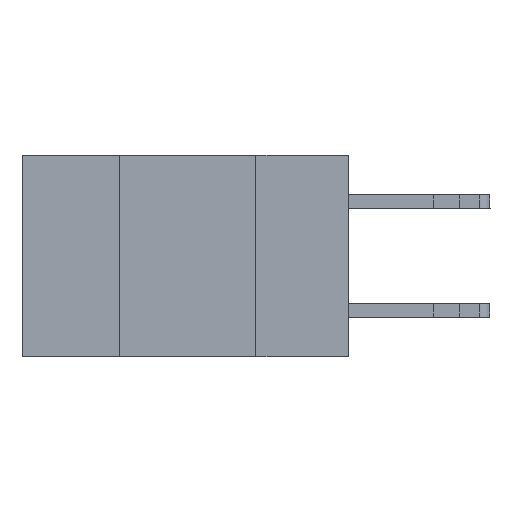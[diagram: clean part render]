
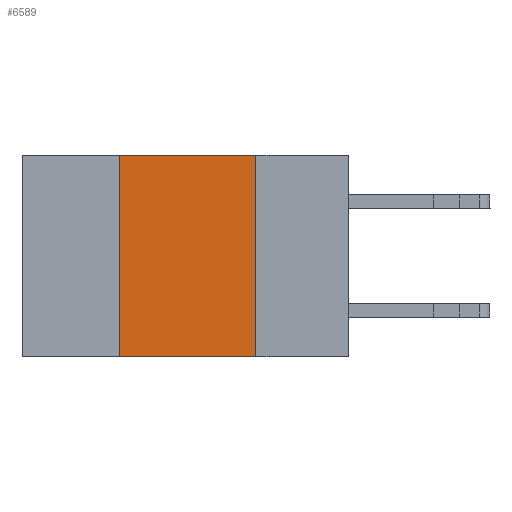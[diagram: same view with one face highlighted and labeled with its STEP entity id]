
A CAD part, left-side view. The second image highlights one B-rep face of the part: STEP entity #6589.
In plain terms, the highlighted planar face has unit normal (-1, 0, 0).
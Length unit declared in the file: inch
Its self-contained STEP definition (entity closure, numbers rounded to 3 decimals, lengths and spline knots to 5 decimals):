
#204 = VERTEX_POINT ( 'NONE', #10092 ) ;
#783 = EDGE_LOOP ( 'NONE', ( #7855, #5674, #4361, #11439 ) ) ;
#1302 = VECTOR ( 'NONE', #2933, 39.37008 ) ;
#1304 = VECTOR ( 'NONE', #6706, 39.37008 ) ;
#1533 = CARTESIAN_POINT ( 'NONE',  ( 0., 0.42, 0. ) ) ;
#2400 = DIRECTION ( 'NONE',  ( 0., 0., -1. ) ) ;
#2801 = EDGE_CURVE ( 'NONE', #14668, #5876, #7875, .T. ) ;
#2933 = DIRECTION ( 'NONE',  ( 0., 0., -1. ) ) ;
#4361 = ORIENTED_EDGE ( 'NONE', *, *, #2801, .F. ) ;
#4415 = FACE_OUTER_BOUND ( 'NONE', #783, .T. ) ;
#5674 = ORIENTED_EDGE ( 'NONE', *, *, #12962, .F. ) ;
#5820 = LINE ( 'NONE', #12784, #6289 ) ;
#5876 = VERTEX_POINT ( 'NONE', #1533 ) ;
#6289 = VECTOR ( 'NONE', #10601, 39.37008 ) ;
#6466 = CARTESIAN_POINT ( 'NONE',  ( 0., 0.17, -0.37 ) ) ;
#6589 = ADVANCED_FACE ( 'NONE', ( #4415 ), #9120, .F. ) ;
#6645 = VECTOR ( 'NONE', #11392, 39.37008 ) ;
#6706 = DIRECTION ( 'NONE',  ( 0., -1., 0. ) ) ;
#6780 = CARTESIAN_POINT ( 'NONE',  ( 0., 0.6, 0. ) ) ;
#6847 = CARTESIAN_POINT ( 'NONE',  ( 0., 0.42, -0.37 ) ) ;
#7727 = CARTESIAN_POINT ( 'NONE',  ( 0., 0.42, -0.37 ) ) ;
#7739 = LINE ( 'NONE', #6780, #1304 ) ;
#7855 = ORIENTED_EDGE ( 'NONE', *, *, #14500, .F. ) ;
#7867 = VERTEX_POINT ( 'NONE', #12275 ) ;
#7875 = LINE ( 'NONE', #6847, #6645 ) ;
#8016 = DIRECTION ( 'NONE',  ( 1., 0., 0. ) ) ;
#9120 = PLANE ( 'NONE',  #13403 ) ;
#10092 = CARTESIAN_POINT ( 'NONE',  ( 0., 0.17, -0.37 ) ) ;
#10601 = DIRECTION ( 'NONE',  ( 0., -1., 0. ) ) ;
#10928 = EDGE_CURVE ( 'NONE', #14668, #204, #5820, .T. ) ;
#11392 = DIRECTION ( 'NONE',  ( 0., 0., 1. ) ) ;
#11439 = ORIENTED_EDGE ( 'NONE', *, *, #10928, .T. ) ;
#12275 = CARTESIAN_POINT ( 'NONE',  ( 0., 0.17, 0. ) ) ;
#12784 = CARTESIAN_POINT ( 'NONE',  ( 0., 0.6, -0.37 ) ) ;
#12962 = EDGE_CURVE ( 'NONE', #5876, #7867, #7739, .T. ) ;
#13403 = AXIS2_PLACEMENT_3D ( 'NONE', #13624, #8016, #2400 ) ;
#13624 = CARTESIAN_POINT ( 'NONE',  ( 0., 0.6, 0. ) ) ;
#14387 = LINE ( 'NONE', #6466, #1302 ) ;
#14500 = EDGE_CURVE ( 'NONE', #7867, #204, #14387, .T. ) ;
#14668 = VERTEX_POINT ( 'NONE', #7727 ) ;
